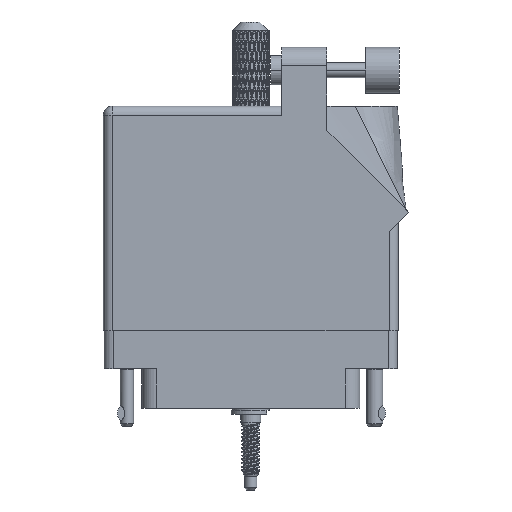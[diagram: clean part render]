
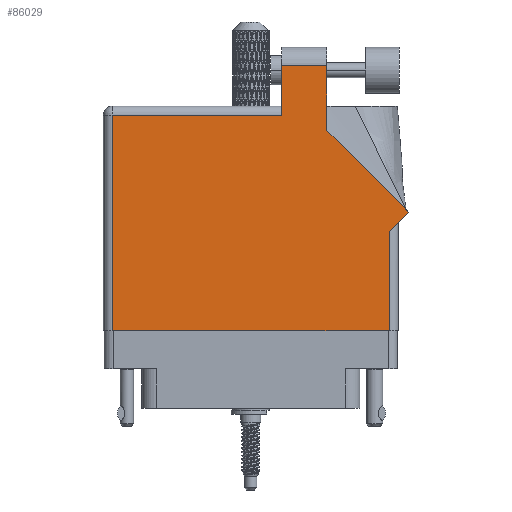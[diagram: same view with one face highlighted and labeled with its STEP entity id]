
A CAD part, front view. The second image highlights one B-rep face of the part: STEP entity #86029.
In plain terms, the highlighted face is planar.
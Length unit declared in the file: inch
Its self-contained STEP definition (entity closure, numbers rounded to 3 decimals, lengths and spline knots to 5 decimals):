
#227 = CARTESIAN_POINT ( 'NONE',  ( 1.217, 1.468, 0. ) ) ;
#295 = DIRECTION ( 'NONE',  ( 0., -1., 0. ) ) ;
#1270 = AXIS2_PLACEMENT_3D ( 'NONE', #102095, #23103, #58301 ) ;
#2013 = EDGE_CURVE ( 'NONE', #12631, #54089, #87365, .T. ) ;
#2383 = ORIENTED_EDGE ( 'NONE', *, *, #53168, .T. ) ;
#6956 = DIRECTION ( 'NONE',  ( 1., 0., 0. ) ) ;
#7492 = CARTESIAN_POINT ( 'NONE',  ( 2.01, 0.737, 0. ) ) ;
#10720 = EDGE_CURVE ( 'NONE', #94209, #54673, #100530, .T. ) ;
#10898 = ORIENTED_EDGE ( 'NONE', *, *, #10720, .T. ) ;
#12590 = DIRECTION ( 'NONE',  ( -1., 0., 0. ) ) ;
#12631 = VERTEX_POINT ( 'NONE', #96449 ) ;
#13931 = LINE ( 'NONE', #49151, #42650 ) ;
#15549 = DIRECTION ( 'NONE',  ( 0.707, 0.707, 0. ) ) ;
#17630 = DIRECTION ( 'NONE',  ( 0., 1., 0. ) ) ;
#19856 = ORIENTED_EDGE ( 'NONE', *, *, #26254, .T. ) ;
#20690 = LINE ( 'NONE', #105664, #44068 ) ;
#23103 = DIRECTION ( 'NONE',  ( 0., 0., -1. ) ) ;
#26254 = EDGE_CURVE ( 'NONE', #62185, #94209, #13931, .T. ) ;
#26883 = CARTESIAN_POINT ( 'NONE',  ( 1.948, 0.737, 0. ) ) ;
#28815 = CARTESIAN_POINT ( 'NONE',  ( 1.524, 1.36442, 0. ) ) ;
#30305 = CARTESIAN_POINT ( 'NONE',  ( 1.948, 0.675, 0. ) ) ;
#31229 = VECTOR ( 'NONE', #70277, 39.37008 ) ;
#31511 = EDGE_CURVE ( 'NONE', #104744, #62185, #68649, .T. ) ;
#31767 = LINE ( 'NONE', #49117, #65394 ) ;
#35079 = CARTESIAN_POINT ( 'NONE',  ( 0., 1.468, 0. ) ) ;
#39105 = ORIENTED_EDGE ( 'NONE', *, *, #73482, .T. ) ;
#42284 = VECTOR ( 'NONE', #295, 39.37008 ) ;
#42650 = VECTOR ( 'NONE', #94653, 39.37008 ) ;
#44068 = VECTOR ( 'NONE', #12590, 39.37008 ) ;
#47741 = VECTOR ( 'NONE', #64633, 39.37008 ) ;
#49117 = CARTESIAN_POINT ( 'NONE',  ( 0., 0., 0. ) ) ;
#49151 = CARTESIAN_POINT ( 'NONE',  ( 2.08071, 0.80771, 0. ) ) ;
#52590 = CARTESIAN_POINT ( 'NONE',  ( 2.08071, 0.80771, 0. ) ) ;
#53168 = EDGE_CURVE ( 'NONE', #54089, #71869, #31767, .T. ) ;
#54089 = VERTEX_POINT ( 'NONE', #72952 ) ;
#54673 = VERTEX_POINT ( 'NONE', #97445 ) ;
#58301 = DIRECTION ( 'NONE',  ( -1., 0., 0. ) ) ;
#61506 = LINE ( 'NONE', #26883, #70116 ) ;
#61950 = ORIENTED_EDGE ( 'NONE', *, *, #107840, .T. ) ;
#62185 = VERTEX_POINT ( 'NONE', #52590 ) ;
#64633 = DIRECTION ( 'NONE',  ( 0., -1., 0. ) ) ;
#64913 = VECTOR ( 'NONE', #15549, 39.37008 ) ;
#65394 = VECTOR ( 'NONE', #6956, 39.37008 ) ;
#66182 = ORIENTED_EDGE ( 'NONE', *, *, #74852, .T. ) ;
#66965 = FACE_OUTER_BOUND ( 'NONE', #112425, .T. ) ;
#68587 = CARTESIAN_POINT ( 'NONE',  ( 1.217, 1.805, 0. ) ) ;
#68649 = LINE ( 'NONE', #7492, #64913 ) ;
#70116 = VECTOR ( 'NONE', #17630, 39.37008 ) ;
#70277 = DIRECTION ( 'NONE',  ( -1., 0., 0. ) ) ;
#71869 = VERTEX_POINT ( 'NONE', #93886 ) ;
#72952 = CARTESIAN_POINT ( 'NONE',  ( 0.062, 0., 0. ) ) ;
#73482 = EDGE_CURVE ( 'NONE', #79008, #12631, #114071, .T. ) ;
#74852 = EDGE_CURVE ( 'NONE', #71869, #104744, #61506, .T. ) ;
#75778 = EDGE_CURVE ( 'NONE', #104469, #79008, #99797, .T. ) ;
#77093 = ORIENTED_EDGE ( 'NONE', *, *, #2013, .T. ) ;
#78170 = CARTESIAN_POINT ( 'NONE',  ( 0.062, 0., 0. ) ) ;
#79008 = VERTEX_POINT ( 'NONE', #227 ) ;
#83826 = CARTESIAN_POINT ( 'NONE',  ( 1.524, 1.36442, 0. ) ) ;
#84751 = VECTOR ( 'NONE', #109162, 39.37008 ) ;
#85416 = ORIENTED_EDGE ( 'NONE', *, *, #75778, .T. ) ;
#86029 = ADVANCED_FACE ( 'NONE', ( #66965 ), #93456, .F. ) ;
#87365 = LINE ( 'NONE', #78170, #42284 ) ;
#93086 = ORIENTED_EDGE ( 'NONE', *, *, #31511, .T. ) ;
#93456 = PLANE ( 'NONE',  #1270 ) ;
#93886 = CARTESIAN_POINT ( 'NONE',  ( 1.948, 0., 0. ) ) ;
#94209 = VERTEX_POINT ( 'NONE', #28815 ) ;
#94653 = DIRECTION ( 'NONE',  ( -0.707, 0.707, 0. ) ) ;
#96449 = CARTESIAN_POINT ( 'NONE',  ( 0.062, 1.468, 0. ) ) ;
#97445 = CARTESIAN_POINT ( 'NONE',  ( 1.524, 1.805, 0. ) ) ;
#99221 = CARTESIAN_POINT ( 'NONE',  ( 1.217, 1.53, 0. ) ) ;
#99797 = LINE ( 'NONE', #99221, #47741 ) ;
#100530 = LINE ( 'NONE', #83826, #84751 ) ;
#102095 = CARTESIAN_POINT ( 'NONE',  ( 0., 1.53, 0. ) ) ;
#104469 = VERTEX_POINT ( 'NONE', #68587 ) ;
#104744 = VERTEX_POINT ( 'NONE', #30305 ) ;
#105664 = CARTESIAN_POINT ( 'NONE',  ( 1.217, 1.805, 0. ) ) ;
#107840 = EDGE_CURVE ( 'NONE', #54673, #104469, #20690, .T. ) ;
#109162 = DIRECTION ( 'NONE',  ( 0., 1., 0. ) ) ;
#112425 = EDGE_LOOP ( 'NONE', ( #10898, #61950, #85416, #39105, #77093, #2383, #66182, #93086, #19856 ) ) ;
#114071 = LINE ( 'NONE', #35079, #31229 ) ;
